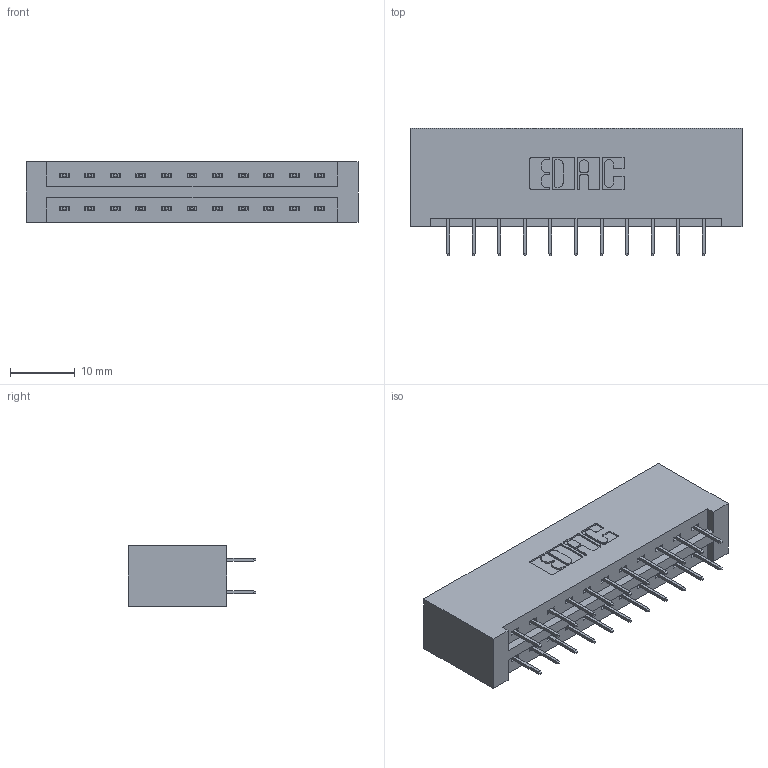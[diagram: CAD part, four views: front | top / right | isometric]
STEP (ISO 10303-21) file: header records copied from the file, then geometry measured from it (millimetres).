
FILE_DESCRIPTION (( 'STEP AP203' ), '1' );
FILE_NAME ('387-022-524-201.STEP', '2019-10-16T16:32:25', ( '' ), ( '' ), 'SwSTEP 2.0', 'SolidWorks 2016', '' );
FILE_SCHEMA (( 'CONFIG_CONTROL_DESIGN' ));
Length unit declared in the file: inch
Products named in the file (3): 387-022-524-201; 345-292-001_345-293-124; 337 Part_No Mounting Lugs
Assembly tree (23 placements, depth 2):
  387-022-524-201
    337 Part_No Mounting Lugs
    345-292-001_345-293-124  x22
Bounding box: 51.46 x 19.69 x 9.4 mm (x, y, z)
Volume: 5738.1 mm3; surface area: 6138.8 mm2
Topology: 23 solids, 23 shells, 1382 faces, 3917 edges, 2522 vertices
Faces by surface type: plane 1034, cylinder 348
Entity records: 12335 total; most frequent: CARTESIAN_POINT 2102, ORIENTED_EDGE 2038, DIRECTION 1839, EDGE_CURVE 1019, VECTOR 903, LINE 903, VERTEX_POINT 674, AXIS2_PLACEMENT_3D 468
